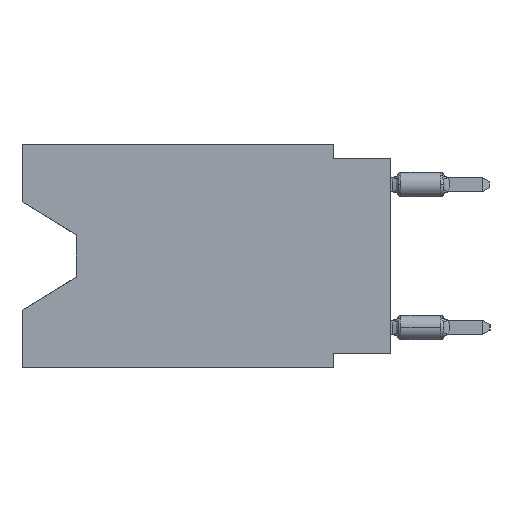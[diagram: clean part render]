
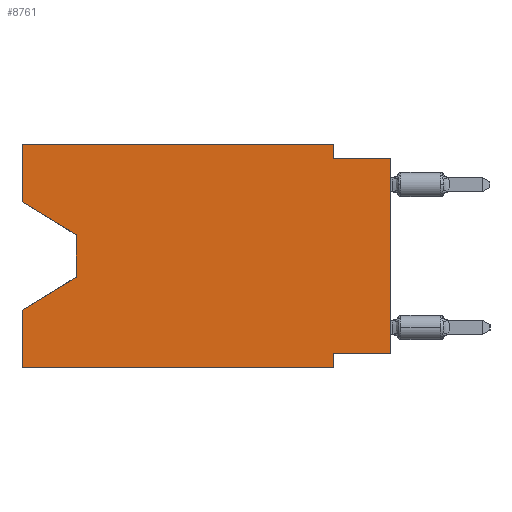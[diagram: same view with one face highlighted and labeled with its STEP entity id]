
A CAD part, left-side view. The second image highlights one B-rep face of the part: STEP entity #8761.
In plain terms, the highlighted planar face has unit normal (-1, 0, 0).
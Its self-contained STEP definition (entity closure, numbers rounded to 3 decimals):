
#122 = EDGE_CURVE ( 'NONE', #50685, #48346, #17439, .T. ) ;
#1842 = VECTOR ( 'NONE', #27856, 1000. ) ;
#2012 = EDGE_CURVE ( 'NONE', #25180, #9050, #10932, .T. ) ;
#2217 = ORIENTED_EDGE ( 'NONE', *, *, #122, .F. ) ;
#5255 = CARTESIAN_POINT ( 'NONE',  ( 0., 2.54, -9.906 ) ) ;
#5431 = ORIENTED_EDGE ( 'NONE', *, *, #38884, .F. ) ;
#5805 = PLANE ( 'NONE',  #26878 ) ;
#6519 = EDGE_CURVE ( 'NONE', #41577, #25180, #22430, .T. ) ;
#6565 = ORIENTED_EDGE ( 'NONE', *, *, #49448, .F. ) ;
#7092 = CARTESIAN_POINT ( 'NONE',  ( 0., 0., -0.635 ) ) ;
#7419 = VERTEX_POINT ( 'NONE', #43589 ) ;
#7763 = CARTESIAN_POINT ( 'NONE',  ( 0., 13.97, -4.013 ) ) ;
#7843 = CARTESIAN_POINT ( 'NONE',  ( 0., 2.54, -0.635 ) ) ;
#8759 = LINE ( 'NONE', #40098, #30913 ) ;
#8761 = ADVANCED_FACE ( 'NONE', ( #33041 ), #5805, .F. ) ;
#8941 = CARTESIAN_POINT ( 'NONE',  ( 0., 16.383, 0. ) ) ;
#9050 = VERTEX_POINT ( 'NONE', #47746 ) ;
#9109 = ORIENTED_EDGE ( 'NONE', *, *, #2012, .T. ) ;
#9152 = DIRECTION ( 'NONE',  ( 1., 0., 0. ) ) ;
#9953 = CARTESIAN_POINT ( 'NONE',  ( 0., 16.383, 0. ) ) ;
#10438 = ORIENTED_EDGE ( 'NONE', *, *, #26509, .T. ) ;
#10932 = LINE ( 'NONE', #30212, #15194 ) ;
#12177 = EDGE_CURVE ( 'NONE', #26763, #7419, #17886, .T. ) ;
#13273 = LINE ( 'NONE', #9953, #28914 ) ;
#13469 = CARTESIAN_POINT ( 'NONE',  ( 0., 16.383, -2.546 ) ) ;
#14187 = ORIENTED_EDGE ( 'NONE', *, *, #43500, .T. ) ;
#14372 = CARTESIAN_POINT ( 'NONE',  ( 0., 0., -9.271 ) ) ;
#15194 = VECTOR ( 'NONE', #45608, 1000. ) ;
#16034 = CARTESIAN_POINT ( 'NONE',  ( 0., 16.383, -9.906 ) ) ;
#16658 = VECTOR ( 'NONE', #46473, 1000. ) ;
#16892 = EDGE_CURVE ( 'NONE', #21507, #42754, #13273, .T. ) ;
#16939 = EDGE_LOOP ( 'NONE', ( #10438, #28813, #9109, #5431, #14187, #6565, #2217, #43114, #43923, #35169, #31744, #48024 ) ) ;
#17339 = CARTESIAN_POINT ( 'NONE',  ( 0., 0., -9.271 ) ) ;
#17439 = LINE ( 'NONE', #14372, #31104 ) ;
#17880 = CARTESIAN_POINT ( 'NONE',  ( 0., 16.383, -2.546 ) ) ;
#17883 = EDGE_CURVE ( 'NONE', #27604, #26763, #34654, .T. ) ;
#17886 = LINE ( 'NONE', #7092, #48984 ) ;
#18351 = CARTESIAN_POINT ( 'NONE',  ( 0., 16.383, 0. ) ) ;
#18705 = CARTESIAN_POINT ( 'NONE',  ( 0., 13.97, -5.893 ) ) ;
#19061 = VECTOR ( 'NONE', #48923, 1000. ) ;
#19672 = DIRECTION ( 'NONE',  ( 0., 1., 0. ) ) ;
#20725 = CARTESIAN_POINT ( 'NONE',  ( 0., 16.383, -9.906 ) ) ;
#21099 = DIRECTION ( 'NONE',  ( 0., 0., 1. ) ) ;
#21507 = VERTEX_POINT ( 'NONE', #13469 ) ;
#21643 = CARTESIAN_POINT ( 'NONE',  ( 0., 0., 0. ) ) ;
#22212 = CARTESIAN_POINT ( 'NONE',  ( 0., 2.54, -9.271 ) ) ;
#22430 = LINE ( 'NONE', #7763, #43831 ) ;
#23999 = VECTOR ( 'NONE', #25494, 1000. ) ;
#24083 = CARTESIAN_POINT ( 'NONE',  ( 0., 2.54, 0. ) ) ;
#25095 = CARTESIAN_POINT ( 'NONE',  ( 0., 16.383, 0. ) ) ;
#25180 = VERTEX_POINT ( 'NONE', #18705 ) ;
#25494 = DIRECTION ( 'NONE',  ( 0., 0., 1. ) ) ;
#25622 = DIRECTION ( 'NONE',  ( 0., 0., 1. ) ) ;
#26407 = VERTEX_POINT ( 'NONE', #20725 ) ;
#26509 = EDGE_CURVE ( 'NONE', #21507, #41577, #29192, .T. ) ;
#26763 = VERTEX_POINT ( 'NONE', #7843 ) ;
#26878 = AXIS2_PLACEMENT_3D ( 'NONE', #25095, #9152, #28936 ) ;
#27604 = VERTEX_POINT ( 'NONE', #24083 ) ;
#27856 = DIRECTION ( 'NONE',  ( 0., -1., 0. ) ) ;
#28813 = ORIENTED_EDGE ( 'NONE', *, *, #6519, .T. ) ;
#28914 = VECTOR ( 'NONE', #25622, 1000. ) ;
#28936 = DIRECTION ( 'NONE',  ( 0., 0., -1. ) ) ;
#29192 = LINE ( 'NONE', #17880, #45133 ) ;
#29225 = CARTESIAN_POINT ( 'NONE',  ( 0., 13.97, -4.013 ) ) ;
#30212 = CARTESIAN_POINT ( 'NONE',  ( 0., 13.97, -5.893 ) ) ;
#30485 = DIRECTION ( 'NONE',  ( 0., -1., 0. ) ) ;
#30913 = VECTOR ( 'NONE', #21099, 1000. ) ;
#31104 = VECTOR ( 'NONE', #19672, 1000. ) ;
#31708 = LINE ( 'NONE', #16034, #1842 ) ;
#31744 = ORIENTED_EDGE ( 'NONE', *, *, #48421, .F. ) ;
#33041 = FACE_OUTER_BOUND ( 'NONE', #16939, .T. ) ;
#34504 = DIRECTION ( 'NONE',  ( 0., 0., -1. ) ) ;
#34654 = LINE ( 'NONE', #38006, #16658 ) ;
#35169 = ORIENTED_EDGE ( 'NONE', *, *, #17883, .F. ) ;
#36156 = VERTEX_POINT ( 'NONE', #39664 ) ;
#38006 = CARTESIAN_POINT ( 'NONE',  ( 0., 2.54, 0. ) ) ;
#38884 = EDGE_CURVE ( 'NONE', #26407, #9050, #8759, .T. ) ;
#39664 = CARTESIAN_POINT ( 'NONE',  ( 0., 2.54, -9.906 ) ) ;
#40098 = CARTESIAN_POINT ( 'NONE',  ( 0., 16.383, 0. ) ) ;
#40201 = LINE ( 'NONE', #5255, #45378 ) ;
#41577 = VERTEX_POINT ( 'NONE', #29225 ) ;
#42754 = VERTEX_POINT ( 'NONE', #8941 ) ;
#43114 = ORIENTED_EDGE ( 'NONE', *, *, #48108, .T. ) ;
#43500 = EDGE_CURVE ( 'NONE', #26407, #36156, #31708, .T. ) ;
#43589 = CARTESIAN_POINT ( 'NONE',  ( 0., 0., -0.635 ) ) ;
#43831 = VECTOR ( 'NONE', #34504, 1000. ) ;
#43923 = ORIENTED_EDGE ( 'NONE', *, *, #12177, .F. ) ;
#44562 = DIRECTION ( 'NONE',  ( 0., 0., -1. ) ) ;
#45008 = LINE ( 'NONE', #21643, #23999 ) ;
#45133 = VECTOR ( 'NONE', #48961, 1000. ) ;
#45378 = VECTOR ( 'NONE', #44562, 1000. ) ;
#45608 = DIRECTION ( 'NONE',  ( 0., 0.855, -0.519 ) ) ;
#46473 = DIRECTION ( 'NONE',  ( 0., 0., -1. ) ) ;
#47746 = CARTESIAN_POINT ( 'NONE',  ( 0., 16.383, -7.36 ) ) ;
#48024 = ORIENTED_EDGE ( 'NONE', *, *, #16892, .F. ) ;
#48108 = EDGE_CURVE ( 'NONE', #50685, #7419, #45008, .T. ) ;
#48346 = VERTEX_POINT ( 'NONE', #22212 ) ;
#48421 = EDGE_CURVE ( 'NONE', #42754, #27604, #48659, .T. ) ;
#48659 = LINE ( 'NONE', #18351, #19061 ) ;
#48923 = DIRECTION ( 'NONE',  ( 0., -1., 0. ) ) ;
#48961 = DIRECTION ( 'NONE',  ( 0., -0.855, -0.519 ) ) ;
#48984 = VECTOR ( 'NONE', #30485, 1000. ) ;
#49448 = EDGE_CURVE ( 'NONE', #48346, #36156, #40201, .T. ) ;
#50685 = VERTEX_POINT ( 'NONE', #17339 ) ;
